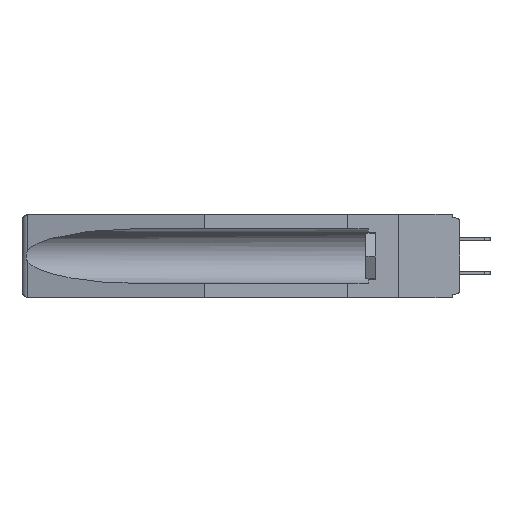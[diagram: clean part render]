
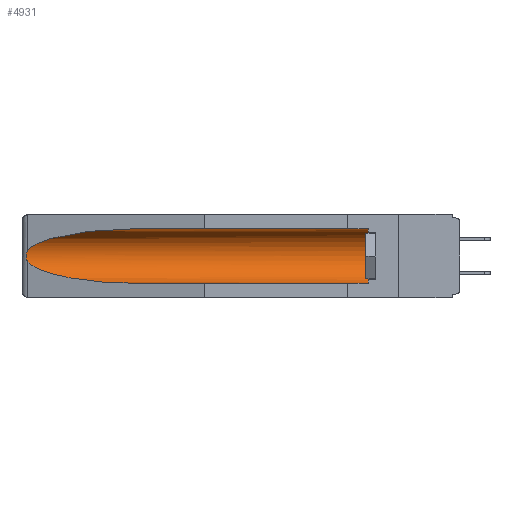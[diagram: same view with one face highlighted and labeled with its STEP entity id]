
A CAD part, left-side view. The second image highlights one B-rep face of the part: STEP entity #4931.
In plain terms, the highlighted cylindrical face has radius 2.857 mm (diameter 5.715 mm), a partial arc.
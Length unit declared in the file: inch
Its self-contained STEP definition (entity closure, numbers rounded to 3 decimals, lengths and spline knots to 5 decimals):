
#73 = ORIENTED_EDGE ( 'NONE', *, *, #8987, .T. ) ;
#81 = CARTESIAN_POINT ( 'NONE',  ( 0.26537, 1.52718, -0.14972 ) ) ;
#1534 = DIRECTION ( 'NONE',  ( 0., 0., 1. ) ) ;
#2615 = CARTESIAN_POINT ( 'NONE',  ( 0.26654, 1.53092, -0.15636 ) ) ;
#3023 = FACE_OUTER_BOUND ( 'NONE', #3682, .T. ) ;
#3682 = EDGE_LOOP ( 'NONE', ( #4113, #7207, #17307, #7542, #73, #16266 ) ) ;
#4113 = ORIENTED_EDGE ( 'NONE', *, *, #17390, .T. ) ;
#4471 = CARTESIAN_POINT ( 'NONE',  ( 0.26537, 1.52718, -0.19328 ) ) ;
#4637 = VERTEX_POINT ( 'NONE', #13713 ) ;
#4931 = ADVANCED_FACE ( 'NONE', ( #3023 ), #8594, .F. ) ;
#5492 = DIRECTION ( 'NONE',  ( 0., 0., 1. ) ) ;
#6420 = CARTESIAN_POINT ( 'NONE',  ( 0.21114, 1.30732, -0.284 ) ) ;
#6995 = LINE ( 'NONE', #12267, #15269 ) ;
#7207 = ORIENTED_EDGE ( 'NONE', *, *, #19716, .T. ) ;
#7249 = AXIS2_PLACEMENT_3D ( 'NONE', #7793, #17066, #1534 ) ;
#7511 = CARTESIAN_POINT ( 'NONE',  ( 0.26655, 1.53094, -0.18657 ) ) ;
#7542 = ORIENTED_EDGE ( 'NONE', *, *, #8244, .F. ) ;
#7793 = CARTESIAN_POINT ( 'NONE',  ( 0.155, -0.30754, -0.1715 ) ) ;
#8244 = EDGE_CURVE ( 'NONE', #16302, #14462, #6995, .T. ) ;
#8594 = CYLINDRICAL_SURFACE ( 'NONE', #7249, 0.1125 ) ;
#8987 = EDGE_CURVE ( 'NONE', #16302, #14850, #12687, .T. ) ;
#9022 = CARTESIAN_POINT ( 'NONE',  ( 0.26537, 1.52718, -0.14972 ) ) ;
#9262 = CARTESIAN_POINT ( 'NONE',  ( 0.26537, 1.52718, -0.19328 ) ) ;
#9444 = CARTESIAN_POINT ( 'NONE',  ( 0.25451, 1.48313, -0.24835 ) ) ;
#10440 = VERTEX_POINT ( 'NONE', #9262 ) ;
#10657 = VECTOR ( 'NONE', #12226, 39.37008 ) ;
#11503 = AXIS2_PLACEMENT_3D ( 'NONE', #13337, #15115, #5492 ) ;
#11903 = EDGE_CURVE ( 'NONE', #10440, #14462, #16897, .T. ) ;
#12184 = CARTESIAN_POINT ( 'NONE',  ( 0.155, 0.126, -0.284 ) ) ;
#12216 = CARTESIAN_POINT ( 'NONE',  ( 0.155, 0.126, -0.059 ) ) ;
#12226 = DIRECTION ( 'NONE',  ( 0., 1., 0. ) ) ;
#12267 = CARTESIAN_POINT ( 'NONE',  ( 0.155, -0.30754, -0.284 ) ) ;
#12338 = CARTESIAN_POINT ( 'NONE',  ( 0.26597, 1.52961, -0.15275 ) ) ;
#12687 = CIRCLE ( 'NONE', #11503, 0.1125 ) ;
#13337 = CARTESIAN_POINT ( 'NONE',  ( 0.155, 0.126, -0.1715 ) ) ;
#13354 = EDGE_CURVE ( 'NONE', #14850, #4637, #14944, .T. ) ;
#13629 = CARTESIAN_POINT ( 'NONE',  ( 0.155, -0.30754, -0.059 ) ) ;
#13713 = CARTESIAN_POINT ( 'NONE',  ( 0.155, 1.07973, -0.059 ) ) ;
#13875 = CARTESIAN_POINT ( 'NONE',  ( 0.2675, 1.53308, -0.16763 ) ) ;
#14111 = CARTESIAN_POINT ( 'NONE',  ( 0.155, 1.07973, -0.284 ) ) ;
#14462 = VERTEX_POINT ( 'NONE', #14111 ) ;
#14847 = CARTESIAN_POINT ( 'NONE',  ( 0.155, 1.07973, -0.059 ) ) ;
#14850 = VERTEX_POINT ( 'NONE', #12216 ) ;
#14941 = B_SPLINE_CURVE_WITH_KNOTS ( 'NONE', 3,
 ( #18666, #12338, #2615, #18867, #13875, #15499, #17110, #7511, #20295, #4471 ),
 .UNSPECIFIED., .F., .F.,
 ( 4, 2, 2, 2, 4 ),
 ( 0., 0.00029, 0.00058, 0.00087, 0.00117 ),
 .UNSPECIFIED. ) ;
#14944 = LINE ( 'NONE', #13629, #10657 ) ;
#15115 = DIRECTION ( 'NONE',  ( 0., -1., 0. ) ) ;
#15269 = VECTOR ( 'NONE', #18932, 39.37008 ) ;
#15499 = CARTESIAN_POINT ( 'NONE',  ( 0.2675, 1.53308, -0.17534 ) ) ;
#16266 = ORIENTED_EDGE ( 'NONE', *, *, #13354, .T. ) ;
#16302 = VERTEX_POINT ( 'NONE', #12184 ) ;
#16897 =( BOUNDED_CURVE ( )  B_SPLINE_CURVE ( 3, ( #17505, #9444, #6420, #17650 ),
 .UNSPECIFIED., .F., .F. ) 
 B_SPLINE_CURVE_WITH_KNOTS ( ( 4, 4 ),
 ( 0.1948, 1.5708 ),
 .UNSPECIFIED. ) 
 CURVE ( )  GEOMETRIC_REPRESENTATION_ITEM ( )  RATIONAL_B_SPLINE_CURVE ( ( 1., 0.848, 0.848, 1. ) ) 
 REPRESENTATION_ITEM ( '' )  );
#17066 = DIRECTION ( 'NONE',  ( 0., 1., 0. ) ) ;
#17110 = CARTESIAN_POINT ( 'NONE',  ( 0.2673, 1.53269, -0.17917 ) ) ;
#17307 = ORIENTED_EDGE ( 'NONE', *, *, #11903, .T. ) ;
#17390 = EDGE_CURVE ( 'NONE', #4637, #17704, #17522, .T. ) ;
#17505 = CARTESIAN_POINT ( 'NONE',  ( 0.26537, 1.52718, -0.19328 ) ) ;
#17522 =( BOUNDED_CURVE ( )  B_SPLINE_CURVE ( 3, ( #14847, #17986, #19470, #81 ),
 .UNSPECIFIED., .F., .F. ) 
 B_SPLINE_CURVE_WITH_KNOTS ( ( 4, 4 ),
 ( 4.71239, 6.08839 ),
 .UNSPECIFIED. ) 
 CURVE ( )  GEOMETRIC_REPRESENTATION_ITEM ( )  RATIONAL_B_SPLINE_CURVE ( ( 1., 0.848, 0.848, 1. ) ) 
 REPRESENTATION_ITEM ( '' )  );
#17650 = CARTESIAN_POINT ( 'NONE',  ( 0.155, 1.07973, -0.284 ) ) ;
#17704 = VERTEX_POINT ( 'NONE', #9022 ) ;
#17986 = CARTESIAN_POINT ( 'NONE',  ( 0.21114, 1.30732, -0.059 ) ) ;
#18666 = CARTESIAN_POINT ( 'NONE',  ( 0.26537, 1.52718, -0.14972 ) ) ;
#18867 = CARTESIAN_POINT ( 'NONE',  ( 0.2673, 1.5327, -0.16383 ) ) ;
#18932 = DIRECTION ( 'NONE',  ( 0., 1., 0. ) ) ;
#19470 = CARTESIAN_POINT ( 'NONE',  ( 0.25451, 1.48313, -0.09465 ) ) ;
#19716 = EDGE_CURVE ( 'NONE', #17704, #10440, #14941, .T. ) ;
#20295 = CARTESIAN_POINT ( 'NONE',  ( 0.26597, 1.5296, -0.19026 ) ) ;
